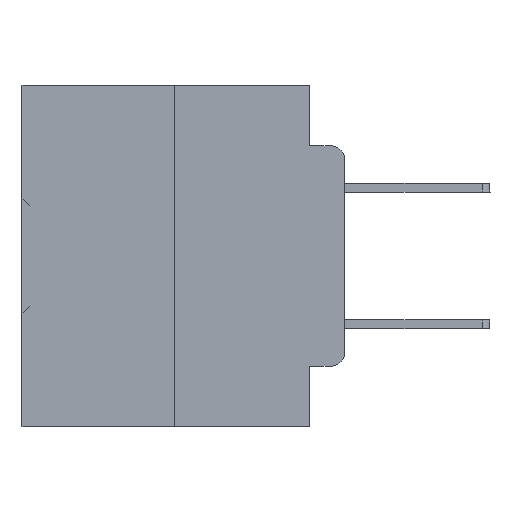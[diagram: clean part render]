
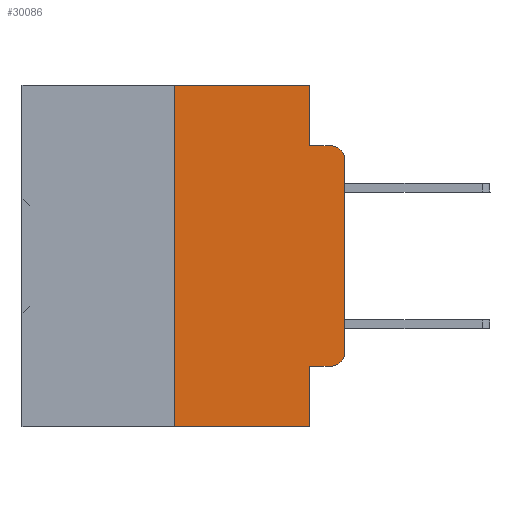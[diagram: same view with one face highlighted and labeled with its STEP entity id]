
A CAD part, left-side view. The second image highlights one B-rep face of the part: STEP entity #30086.
In plain terms, the highlighted planar face has unit normal (-1, 0, 0).
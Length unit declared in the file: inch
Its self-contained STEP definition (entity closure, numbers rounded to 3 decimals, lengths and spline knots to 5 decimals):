
#452 = ORIENTED_EDGE ( 'NONE', *, *, #25111, .F. ) ;
#526 = VECTOR ( 'NONE', #28272, 39.37008 ) ;
#541 = CARTESIAN_POINT ( 'NONE',  ( 0., 0.25, 0. ) ) ;
#1108 = CARTESIAN_POINT ( 'NONE',  ( 0., 0.473, 0. ) ) ;
#1367 = PLANE ( 'NONE',  #4957 ) ;
#1812 = CIRCLE ( 'NONE', #6832, 0.02 ) ;
#2631 = CARTESIAN_POINT ( 'NONE',  ( 0., 0., 0. ) ) ;
#2769 = DIRECTION ( 'NONE',  ( 0., -1., 0. ) ) ;
#3280 = FACE_OUTER_BOUND ( 'NONE', #25405, .T. ) ;
#4001 = ORIENTED_EDGE ( 'NONE', *, *, #37348, .F. ) ;
#4343 = DIRECTION ( 'NONE',  ( 0., -1., 0. ) ) ;
#4595 = CARTESIAN_POINT ( 'NONE',  ( 0., 0.473, 0. ) ) ;
#4957 = AXIS2_PLACEMENT_3D ( 'NONE', #4595, #26215, #7757 ) ;
#6272 = VERTEX_POINT ( 'NONE', #33644 ) ;
#6762 = CARTESIAN_POINT ( 'NONE',  ( 0., 0.051, 0. ) ) ;
#6832 = AXIS2_PLACEMENT_3D ( 'NONE', #17546, #38847, #20657 ) ;
#6977 = VERTEX_POINT ( 'NONE', #25356 ) ;
#7093 = LINE ( 'NONE', #1108, #31619 ) ;
#7311 = CARTESIAN_POINT ( 'NONE',  ( 0., 0.25, -0.5 ) ) ;
#7757 = DIRECTION ( 'NONE',  ( 0., 0., -1. ) ) ;
#8323 = VECTOR ( 'NONE', #16491, 39.37008 ) ;
#9083 = VECTOR ( 'NONE', #2769, 39.37008 ) ;
#9274 = LINE ( 'NONE', #13343, #8323 ) ;
#9870 = EDGE_CURVE ( 'NONE', #27042, #30036, #16285, .T. ) ;
#11835 = ORIENTED_EDGE ( 'NONE', *, *, #21077, .T. ) ;
#11909 = CARTESIAN_POINT ( 'NONE',  ( 0., 0.02, -0.1085 ) ) ;
#11954 = EDGE_CURVE ( 'NONE', #19928, #27042, #24121, .T. ) ;
#12067 = DIRECTION ( 'NONE',  ( 0., 0., 1. ) ) ;
#12304 = LINE ( 'NONE', #39931, #19613 ) ;
#13343 = CARTESIAN_POINT ( 'NONE',  ( 0., 0.051, 0. ) ) ;
#13551 = EDGE_CURVE ( 'NONE', #22141, #6272, #7093, .T. ) ;
#14250 = ORIENTED_EDGE ( 'NONE', *, *, #13551, .F. ) ;
#14619 = LINE ( 'NONE', #18399, #21888 ) ;
#15027 = DIRECTION ( 'NONE',  ( 0., 0., -1. ) ) ;
#15939 = VECTOR ( 'NONE', #12067, 39.37008 ) ;
#16087 = CARTESIAN_POINT ( 'NONE',  ( 0., 0.25, 0. ) ) ;
#16196 = ORIENTED_EDGE ( 'NONE', *, *, #33255, .F. ) ;
#16285 = CIRCLE ( 'NONE', #37513, 0.02 ) ;
#16491 = DIRECTION ( 'NONE',  ( 0., 0., -1. ) ) ;
#17546 = CARTESIAN_POINT ( 'NONE',  ( 0., 0.02, -0.3915 ) ) ;
#17791 = VERTEX_POINT ( 'NONE', #7311 ) ;
#18340 = CARTESIAN_POINT ( 'NONE',  ( 0., 0.051, -0.4115 ) ) ;
#18399 = CARTESIAN_POINT ( 'NONE',  ( 0., 0.051, -0.0885 ) ) ;
#18748 = EDGE_CURVE ( 'NONE', #17791, #6977, #12304, .T. ) ;
#19587 = VERTEX_POINT ( 'NONE', #25517 ) ;
#19613 = VECTOR ( 'NONE', #36881, 39.37008 ) ;
#19928 = VERTEX_POINT ( 'NONE', #26959 ) ;
#20577 = ORIENTED_EDGE ( 'NONE', *, *, #35330, .F. ) ;
#20657 = DIRECTION ( 'NONE',  ( 0., 0., -1. ) ) ;
#21077 = EDGE_CURVE ( 'NONE', #27583, #19928, #1812, .T. ) ;
#21888 = VECTOR ( 'NONE', #36649, 39.37008 ) ;
#22141 = VERTEX_POINT ( 'NONE', #541 ) ;
#22859 = CARTESIAN_POINT ( 'NONE',  ( 0., 0., -0.1085 ) ) ;
#22925 = ORIENTED_EDGE ( 'NONE', *, *, #11954, .T. ) ;
#22963 = LINE ( 'NONE', #6762, #37235 ) ;
#23078 = EDGE_CURVE ( 'NONE', #35121, #27583, #33581, .T. ) ;
#24121 = LINE ( 'NONE', #2631, #15939 ) ;
#25111 = EDGE_CURVE ( 'NONE', #35121, #6977, #22963, .T. ) ;
#25356 = CARTESIAN_POINT ( 'NONE',  ( 0., 0.051, -0.5 ) ) ;
#25405 = EDGE_LOOP ( 'NONE', ( #22925, #27682, #4001, #20577, #14250, #16196, #32469, #452, #35339, #11835 ) ) ;
#25474 = CARTESIAN_POINT ( 'NONE',  ( 0., 0.02, -0.4115 ) ) ;
#25517 = CARTESIAN_POINT ( 'NONE',  ( 0., 0.051, -0.0885 ) ) ;
#25940 = CARTESIAN_POINT ( 'NONE',  ( 0., 0.02, -0.0885 ) ) ;
#26215 = DIRECTION ( 'NONE',  ( 1., 0., 0. ) ) ;
#26959 = CARTESIAN_POINT ( 'NONE',  ( 0., 0., -0.3915 ) ) ;
#27042 = VERTEX_POINT ( 'NONE', #22859 ) ;
#27583 = VERTEX_POINT ( 'NONE', #25474 ) ;
#27682 = ORIENTED_EDGE ( 'NONE', *, *, #9870, .T. ) ;
#27744 = CARTESIAN_POINT ( 'NONE',  ( 0., 0.051, -0.4115 ) ) ;
#28272 = DIRECTION ( 'NONE',  ( 0., 0., 1. ) ) ;
#28285 = DIRECTION ( 'NONE',  ( 0., 0., -1. ) ) ;
#30036 = VERTEX_POINT ( 'NONE', #25940 ) ;
#30086 = ADVANCED_FACE ( 'NONE', ( #3280 ), #1367, .F. ) ;
#31619 = VECTOR ( 'NONE', #4343, 39.37008 ) ;
#32469 = ORIENTED_EDGE ( 'NONE', *, *, #18748, .T. ) ;
#32529 = LINE ( 'NONE', #16087, #526 ) ;
#33255 = EDGE_CURVE ( 'NONE', #17791, #22141, #32529, .T. ) ;
#33343 = DIRECTION ( 'NONE',  ( -1., 0., 0. ) ) ;
#33581 = LINE ( 'NONE', #18340, #9083 ) ;
#33644 = CARTESIAN_POINT ( 'NONE',  ( 0., 0.051, 0. ) ) ;
#35121 = VERTEX_POINT ( 'NONE', #27744 ) ;
#35330 = EDGE_CURVE ( 'NONE', #6272, #19587, #9274, .T. ) ;
#35339 = ORIENTED_EDGE ( 'NONE', *, *, #23078, .T. ) ;
#36649 = DIRECTION ( 'NONE',  ( 0., -1., 0. ) ) ;
#36881 = DIRECTION ( 'NONE',  ( 0., -1., 0. ) ) ;
#37235 = VECTOR ( 'NONE', #28285, 39.37008 ) ;
#37348 = EDGE_CURVE ( 'NONE', #19587, #30036, #14619, .T. ) ;
#37513 = AXIS2_PLACEMENT_3D ( 'NONE', #11909, #33343, #15027 ) ;
#38847 = DIRECTION ( 'NONE',  ( -1., 0., 0. ) ) ;
#39931 = CARTESIAN_POINT ( 'NONE',  ( 0., 0.473, -0.5 ) ) ;
